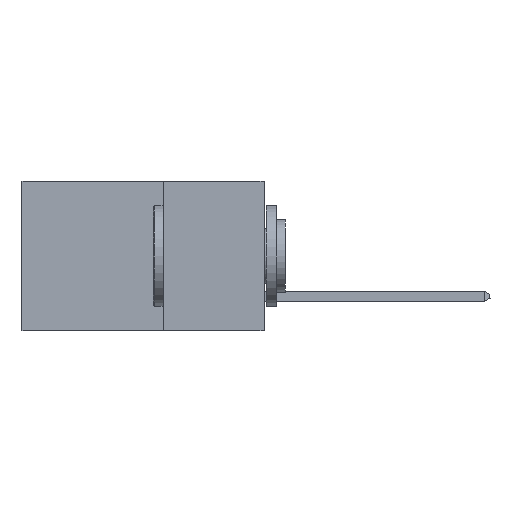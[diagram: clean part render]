
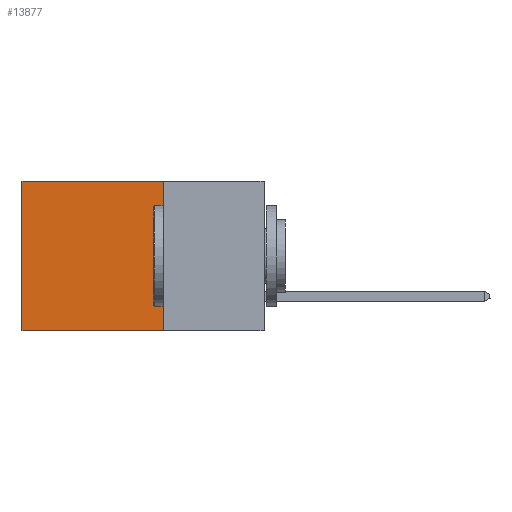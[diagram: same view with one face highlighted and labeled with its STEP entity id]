
A CAD part, left-side view. The second image highlights one B-rep face of the part: STEP entity #13877.
In plain terms, the highlighted planar face has unit normal (-1, 0, 0).
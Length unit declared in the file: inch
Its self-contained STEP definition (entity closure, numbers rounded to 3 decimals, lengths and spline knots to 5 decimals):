
#31 = CARTESIAN_POINT ( 'NONE',  ( 0.2615, 0.6, -0.37 ) ) ;
#1344 = DIRECTION ( 'NONE',  ( 0., 0., -1. ) ) ;
#2447 = CARTESIAN_POINT ( 'NONE',  ( 0.2615, 0.25, -0.37 ) ) ;
#2516 = DIRECTION ( 'NONE',  ( 1., 0., 0. ) ) ;
#2628 = LINE ( 'NONE', #14179, #11421 ) ;
#2925 = CARTESIAN_POINT ( 'NONE',  ( 0.2615, 0.6, 0. ) ) ;
#3006 = AXIS2_PLACEMENT_3D ( 'NONE', #11118, #2516, #3688 ) ;
#3125 = VERTEX_POINT ( 'NONE', #5873 ) ;
#3222 = CARTESIAN_POINT ( 'NONE',  ( 0.2615, 0.6, -0.37 ) ) ;
#3297 = ORIENTED_EDGE ( 'NONE', *, *, #8017, .T. ) ;
#3688 = DIRECTION ( 'NONE',  ( 0., 0., -1. ) ) ;
#4576 = LINE ( 'NONE', #2447, #8910 ) ;
#4998 = EDGE_CURVE ( 'NONE', #3125, #9096, #4576, .T. ) ;
#5091 = DIRECTION ( 'NONE',  ( 0., 1., 0. ) ) ;
#5316 = VECTOR ( 'NONE', #5091, 39.37008 ) ;
#5625 = DIRECTION ( 'NONE',  ( 0., 1., 0. ) ) ;
#5873 = CARTESIAN_POINT ( 'NONE',  ( 0.2615, 0.25, 0. ) ) ;
#6149 = EDGE_LOOP ( 'NONE', ( #3297, #6188, #13752, #12893 ) ) ;
#6163 = EDGE_CURVE ( 'NONE', #3125, #11371, #13257, .T. ) ;
#6188 = ORIENTED_EDGE ( 'NONE', *, *, #13114, .F. ) ;
#7072 = FACE_OUTER_BOUND ( 'NONE', #6149, .T. ) ;
#7315 = LINE ( 'NONE', #31, #9765 ) ;
#8017 = EDGE_CURVE ( 'NONE', #11371, #10579, #7315, .T. ) ;
#8910 = VECTOR ( 'NONE', #9160, 39.37008 ) ;
#9096 = VERTEX_POINT ( 'NONE', #14199 ) ;
#9160 = DIRECTION ( 'NONE',  ( 0., 0., -1. ) ) ;
#9505 = CARTESIAN_POINT ( 'NONE',  ( 0.2615, 0.25, 0. ) ) ;
#9765 = VECTOR ( 'NONE', #1344, 39.37008 ) ;
#10579 = VERTEX_POINT ( 'NONE', #3222 ) ;
#11118 = CARTESIAN_POINT ( 'NONE',  ( 0.2615, 0.25, -0.37 ) ) ;
#11371 = VERTEX_POINT ( 'NONE', #2925 ) ;
#11421 = VECTOR ( 'NONE', #5625, 39.37008 ) ;
#12893 = ORIENTED_EDGE ( 'NONE', *, *, #6163, .T. ) ;
#13114 = EDGE_CURVE ( 'NONE', #9096, #10579, #2628, .T. ) ;
#13238 = PLANE ( 'NONE',  #3006 ) ;
#13257 = LINE ( 'NONE', #9505, #5316 ) ;
#13752 = ORIENTED_EDGE ( 'NONE', *, *, #4998, .F. ) ;
#13877 = ADVANCED_FACE ( 'NONE', ( #7072 ), #13238, .F. ) ;
#14179 = CARTESIAN_POINT ( 'NONE',  ( 0.2615, 0.25, -0.37 ) ) ;
#14199 = CARTESIAN_POINT ( 'NONE',  ( 0.2615, 0.25, -0.37 ) ) ;
